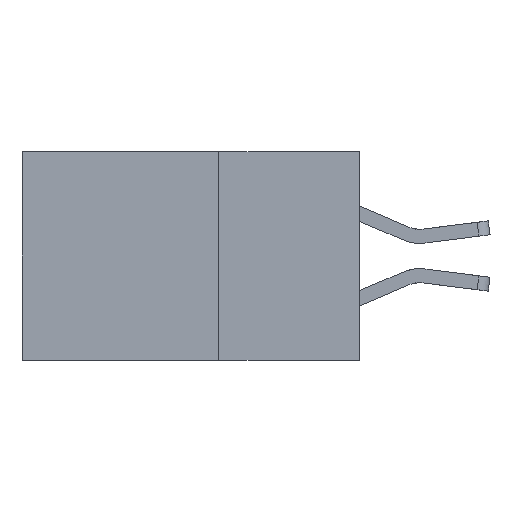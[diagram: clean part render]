
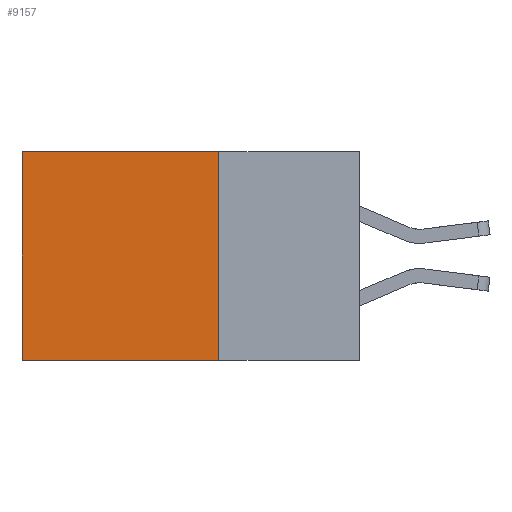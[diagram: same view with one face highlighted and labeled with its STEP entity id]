
A CAD part, left-side view. The second image highlights one B-rep face of the part: STEP entity #9157.
In plain terms, the highlighted planar face has unit normal (-1, 0, 0).
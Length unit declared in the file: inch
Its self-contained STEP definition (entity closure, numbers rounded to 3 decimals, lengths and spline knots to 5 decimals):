
#196 = AXIS2_PLACEMENT_3D ( 'NONE', #1540, #5396, #6704 ) ;
#432 = LINE ( 'NONE', #5833, #1767 ) ;
#477 = LINE ( 'NONE', #2045, #7939 ) ;
#627 = VERTEX_POINT ( 'NONE', #6399 ) ;
#659 = CARTESIAN_POINT ( 'NONE',  ( 0.2875, 0.6, 0. ) ) ;
#717 = PLANE ( 'NONE',  #196 ) ;
#857 = FACE_OUTER_BOUND ( 'NONE', #9130, .T. ) ;
#867 = ORIENTED_EDGE ( 'NONE', *, *, #7919, .F. ) ;
#1476 = DIRECTION ( 'NONE',  ( 0., 1., 0. ) ) ;
#1540 = CARTESIAN_POINT ( 'NONE',  ( 0.2875, 0.25, 0. ) ) ;
#1697 = LINE ( 'NONE', #8416, #2185 ) ;
#1767 = VECTOR ( 'NONE', #1476, 39.37008 ) ;
#1994 = DIRECTION ( 'NONE',  ( 0., 0., -1. ) ) ;
#2045 = CARTESIAN_POINT ( 'NONE',  ( 0.2875, 0.25, 0. ) ) ;
#2185 = VECTOR ( 'NONE', #5364, 39.37008 ) ;
#2212 = EDGE_CURVE ( 'NONE', #3266, #7935, #1697, .T. ) ;
#3266 = VERTEX_POINT ( 'NONE', #3517 ) ;
#3322 = DIRECTION ( 'NONE',  ( 0., 0., -1. ) ) ;
#3517 = CARTESIAN_POINT ( 'NONE',  ( 0.2875, 0.25, 0. ) ) ;
#4162 = EDGE_CURVE ( 'NONE', #3266, #627, #477, .T. ) ;
#4564 = VERTEX_POINT ( 'NONE', #6369 ) ;
#5364 = DIRECTION ( 'NONE',  ( 0., 1., 0. ) ) ;
#5396 = DIRECTION ( 'NONE',  ( 1., 0., 0. ) ) ;
#5733 = ORIENTED_EDGE ( 'NONE', *, *, #2212, .T. ) ;
#5833 = CARTESIAN_POINT ( 'NONE',  ( 0.2875, 0.25, -0.37 ) ) ;
#6369 = CARTESIAN_POINT ( 'NONE',  ( 0.2875, 0.6, -0.37 ) ) ;
#6399 = CARTESIAN_POINT ( 'NONE',  ( 0.2875, 0.25, -0.37 ) ) ;
#6575 = ORIENTED_EDGE ( 'NONE', *, *, #8667, .T. ) ;
#6704 = DIRECTION ( 'NONE',  ( 0., 0., -1. ) ) ;
#7526 = VECTOR ( 'NONE', #3322, 39.37008 ) ;
#7726 = LINE ( 'NONE', #9255, #7526 ) ;
#7919 = EDGE_CURVE ( 'NONE', #627, #4564, #432, .T. ) ;
#7935 = VERTEX_POINT ( 'NONE', #659 ) ;
#7939 = VECTOR ( 'NONE', #1994, 39.37008 ) ;
#8416 = CARTESIAN_POINT ( 'NONE',  ( 0.2875, 0.25, 0. ) ) ;
#8622 = ORIENTED_EDGE ( 'NONE', *, *, #4162, .F. ) ;
#8667 = EDGE_CURVE ( 'NONE', #7935, #4564, #7726, .T. ) ;
#9130 = EDGE_LOOP ( 'NONE', ( #6575, #867, #8622, #5733 ) ) ;
#9157 = ADVANCED_FACE ( 'NONE', ( #857 ), #717, .F. ) ;
#9255 = CARTESIAN_POINT ( 'NONE',  ( 0.2875, 0.6, 0. ) ) ;
